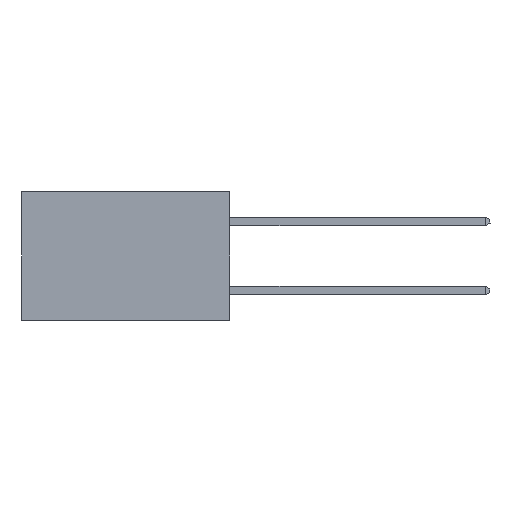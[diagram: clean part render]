
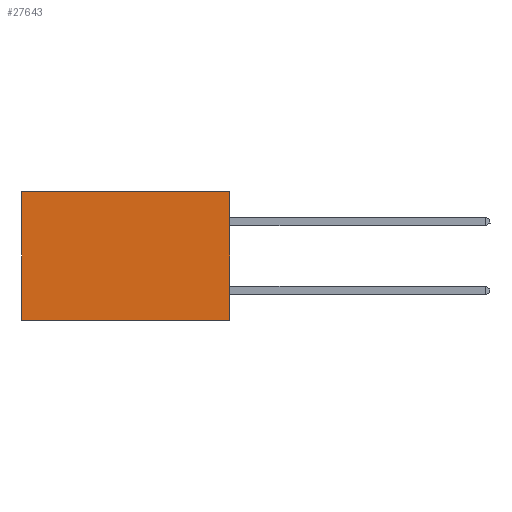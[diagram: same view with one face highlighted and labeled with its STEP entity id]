
A CAD part, left-side view. The second image highlights one B-rep face of the part: STEP entity #27643.
In plain terms, the highlighted planar face has unit normal (-1, 0, 0).
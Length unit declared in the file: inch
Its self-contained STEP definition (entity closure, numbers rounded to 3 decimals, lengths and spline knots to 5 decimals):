
#1378 = CARTESIAN_POINT ( 'NONE',  ( 0.298, 0., -0.37 ) ) ;
#1792 = VERTEX_POINT ( 'NONE', #18994 ) ;
#2768 = LINE ( 'NONE', #20070, #22166 ) ;
#3161 = ORIENTED_EDGE ( 'NONE', *, *, #28683, .T. ) ;
#5534 = ORIENTED_EDGE ( 'NONE', *, *, #11743, .F. ) ;
#6496 = DIRECTION ( 'NONE',  ( 0., 1., 0. ) ) ;
#6754 = DIRECTION ( 'NONE',  ( 1., 0., 0. ) ) ;
#7245 = VECTOR ( 'NONE', #6496, 39.37008 ) ;
#7488 = DIRECTION ( 'NONE',  ( 0., 0., -1. ) ) ;
#8047 = EDGE_CURVE ( 'NONE', #1792, #19643, #13979, .T. ) ;
#9640 = CARTESIAN_POINT ( 'NONE',  ( 0.298, 0., 0. ) ) ;
#10562 = VECTOR ( 'NONE', #13349, 39.37008 ) ;
#10789 = CARTESIAN_POINT ( 'NONE',  ( 0.298, 0., 0. ) ) ;
#11743 = EDGE_CURVE ( 'NONE', #30936, #1792, #30621, .T. ) ;
#11894 = AXIS2_PLACEMENT_3D ( 'NONE', #21903, #6754, #24455 ) ;
#13349 = DIRECTION ( 'NONE',  ( 0., 1., 0. ) ) ;
#13979 = LINE ( 'NONE', #1378, #7245 ) ;
#14278 = PLANE ( 'NONE',  #11894 ) ;
#14743 = CARTESIAN_POINT ( 'NONE',  ( 0.298, 0.6, -0.37 ) ) ;
#16461 = CARTESIAN_POINT ( 'NONE',  ( 0.298, 0.6, 0. ) ) ;
#17754 = FACE_OUTER_BOUND ( 'NONE', #29958, .T. ) ;
#18994 = CARTESIAN_POINT ( 'NONE',  ( 0.298, 0., -0.37 ) ) ;
#19643 = VERTEX_POINT ( 'NONE', #14743 ) ;
#20070 = CARTESIAN_POINT ( 'NONE',  ( 0.298, 0.6, 0. ) ) ;
#21796 = CARTESIAN_POINT ( 'NONE',  ( 0.298, 0., 0. ) ) ;
#21903 = CARTESIAN_POINT ( 'NONE',  ( 0.298, 0., 0. ) ) ;
#22166 = VECTOR ( 'NONE', #7488, 39.37008 ) ;
#22396 = ORIENTED_EDGE ( 'NONE', *, *, #8047, .F. ) ;
#23465 = ORIENTED_EDGE ( 'NONE', *, *, #29785, .T. ) ;
#23904 = VECTOR ( 'NONE', #29452, 39.37008 ) ;
#24455 = DIRECTION ( 'NONE',  ( 0., 0., -1. ) ) ;
#27643 = ADVANCED_FACE ( 'NONE', ( #17754 ), #14278, .F. ) ;
#28683 = EDGE_CURVE ( 'NONE', #30936, #31434, #30736, .T. ) ;
#29452 = DIRECTION ( 'NONE',  ( 0., 0., -1. ) ) ;
#29785 = EDGE_CURVE ( 'NONE', #31434, #19643, #2768, .T. ) ;
#29958 = EDGE_LOOP ( 'NONE', ( #23465, #22396, #5534, #3161 ) ) ;
#30621 = LINE ( 'NONE', #21796, #23904 ) ;
#30736 = LINE ( 'NONE', #10789, #10562 ) ;
#30936 = VERTEX_POINT ( 'NONE', #9640 ) ;
#31434 = VERTEX_POINT ( 'NONE', #16461 ) ;
